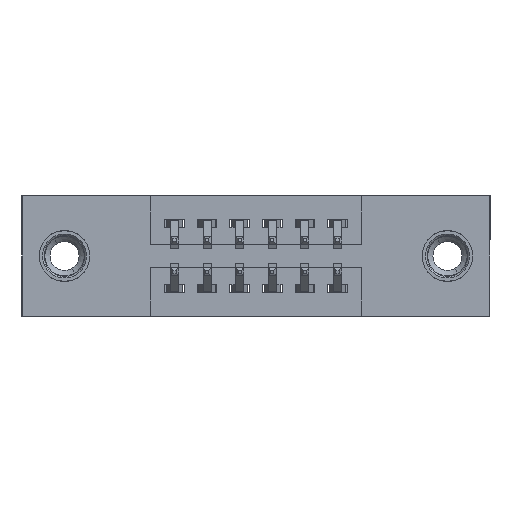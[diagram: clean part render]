
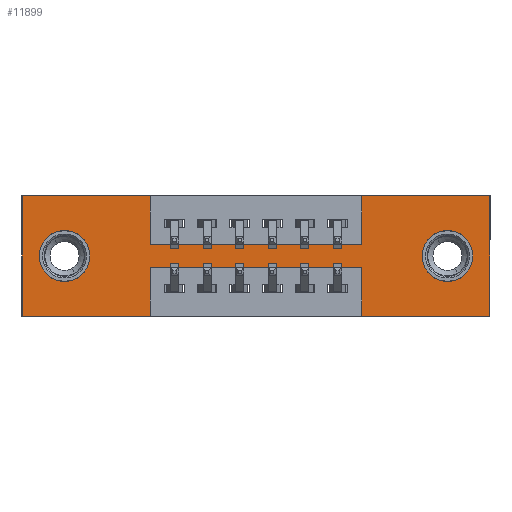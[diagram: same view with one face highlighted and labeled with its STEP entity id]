
A CAD part, front view. The second image highlights one B-rep face of the part: STEP entity #11899.
In plain terms, the highlighted planar face has unit normal (0, -1, 0).
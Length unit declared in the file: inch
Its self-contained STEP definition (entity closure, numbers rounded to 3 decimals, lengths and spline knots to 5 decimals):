
#12 = CARTESIAN_POINT ( 'NONE',  ( 1.0425, 0., -0.22 ) ) ;
#330 = DIRECTION ( 'NONE',  ( 0., -1., 0. ) ) ;
#574 = CARTESIAN_POINT ( 'NONE',  ( 0., 0., 0. ) ) ;
#660 = VECTOR ( 'NONE', #7857, 39.37008 ) ;
#666 = VERTEX_POINT ( 'NONE', #9988 ) ;
#913 = CARTESIAN_POINT ( 'NONE',  ( 0.13, 0., -0.185 ) ) ;
#924 = DIRECTION ( 'NONE',  ( -1., 0., 0. ) ) ;
#960 = EDGE_CURVE ( 'NONE', #5471, #2403, #10943, .T. ) ;
#980 = VERTEX_POINT ( 'NONE', #2272 ) ;
#1102 = EDGE_CURVE ( 'NONE', #11484, #6568, #4636, .T. ) ;
#1441 = DIRECTION ( 'NONE',  ( 0., 0., -1. ) ) ;
#1444 = VERTEX_POINT ( 'NONE', #6535 ) ;
#1849 = DIRECTION ( 'NONE',  ( 0., 0., 1. ) ) ;
#1892 = CARTESIAN_POINT ( 'NONE',  ( 0.3925, 0., -0.37 ) ) ;
#2001 = VECTOR ( 'NONE', #6488, 39.37008 ) ;
#2020 = CARTESIAN_POINT ( 'NONE',  ( 1.0425, 0., -0.37 ) ) ;
#2093 = ORIENTED_EDGE ( 'NONE', *, *, #5328, .F. ) ;
#2225 = EDGE_CURVE ( 'NONE', #10936, #7716, #7904, .T. ) ;
#2272 = CARTESIAN_POINT ( 'NONE',  ( 1.435, 0., 0. ) ) ;
#2368 = VECTOR ( 'NONE', #1441, 39.37008 ) ;
#2403 = VERTEX_POINT ( 'NONE', #3284 ) ;
#2464 = DIRECTION ( 'NONE',  ( 0., 0., 1. ) ) ;
#2514 = EDGE_CURVE ( 'NONE', #2403, #5872, #2651, .T. ) ;
#2546 = CARTESIAN_POINT ( 'NONE',  ( 0.3925, 0., -0.37 ) ) ;
#2635 = CARTESIAN_POINT ( 'NONE',  ( 1.0425, 0., 0. ) ) ;
#2651 = LINE ( 'NONE', #1892, #2368 ) ;
#2683 = CARTESIAN_POINT ( 'NONE',  ( 1.0425, 0., -0.37 ) ) ;
#2715 = AXIS2_PLACEMENT_3D ( 'NONE', #8161, #2724, #9088 ) ;
#2724 = DIRECTION ( 'NONE',  ( 0., 1., 0. ) ) ;
#2740 = EDGE_LOOP ( 'NONE', ( #7379, #7641, #11717, #3860, #4377, #10433, #2093, #8169, #8147, #10145, #6771, #6318 ) ) ;
#2841 = FACE_BOUND ( 'NONE', #7031, .T. ) ;
#2886 = CARTESIAN_POINT ( 'NONE',  ( 1.305, 0., -0.185 ) ) ;
#3093 = VECTOR ( 'NONE', #10019, 39.37008 ) ;
#3133 = LINE ( 'NONE', #9705, #660 ) ;
#3284 = CARTESIAN_POINT ( 'NONE',  ( 0.3925, 0., -0.22 ) ) ;
#3323 = CARTESIAN_POINT ( 'NONE',  ( 1.305, 0., -0.107 ) ) ;
#3369 = AXIS2_PLACEMENT_3D ( 'NONE', #913, #7292, #1849 ) ;
#3458 = EDGE_CURVE ( 'NONE', #10690, #666, #11189, .T. ) ;
#3465 = VERTEX_POINT ( 'NONE', #3323 ) ;
#3495 = CARTESIAN_POINT ( 'NONE',  ( 0., 0., 0. ) ) ;
#3556 = VECTOR ( 'NONE', #11845, 39.37008 ) ;
#3683 = DIRECTION ( 'NONE',  ( 1., 0., 0. ) ) ;
#3703 = ORIENTED_EDGE ( 'NONE', *, *, #6675, .T. ) ;
#3789 = DIRECTION ( 'NONE',  ( 0., 0., -1. ) ) ;
#3831 = VECTOR ( 'NONE', #11718, 39.37008 ) ;
#3860 = ORIENTED_EDGE ( 'NONE', *, *, #5424, .F. ) ;
#3888 = DIRECTION ( 'NONE',  ( 1., 0., 0. ) ) ;
#4115 = EDGE_CURVE ( 'NONE', #6568, #11484, #4578, .T. ) ;
#4146 = CARTESIAN_POINT ( 'NONE',  ( 0.3925, 0., -0.22 ) ) ;
#4232 = CIRCLE ( 'NONE', #10131, 0.078 ) ;
#4377 = ORIENTED_EDGE ( 'NONE', *, *, #4827, .F. ) ;
#4406 = DIRECTION ( 'NONE',  ( 0., 1., 0. ) ) ;
#4578 = CIRCLE ( 'NONE', #3369, 0.078 ) ;
#4636 = CIRCLE ( 'NONE', #6461, 0.078 ) ;
#4687 = LINE ( 'NONE', #5579, #6827 ) ;
#4827 = EDGE_CURVE ( 'NONE', #980, #8665, #4687, .T. ) ;
#4829 = EDGE_CURVE ( 'NONE', #5872, #5750, #9265, .T. ) ;
#4859 = ORIENTED_EDGE ( 'NONE', *, *, #4115, .T. ) ;
#4879 = LINE ( 'NONE', #10794, #11925 ) ;
#4903 = AXIS2_PLACEMENT_3D ( 'NONE', #11338, #330, #6755 ) ;
#4921 = PLANE ( 'NONE',  #4903 ) ;
#5164 = CARTESIAN_POINT ( 'NONE',  ( 1.0425, 0., -0.15 ) ) ;
#5190 = EDGE_CURVE ( 'NONE', #5750, #10690, #3133, .T. ) ;
#5328 = EDGE_CURVE ( 'NONE', #7716, #1444, #11125, .T. ) ;
#5424 = EDGE_CURVE ( 'NONE', #8665, #6189, #5680, .T. ) ;
#5471 = VERTEX_POINT ( 'NONE', #12 ) ;
#5537 = VERTEX_POINT ( 'NONE', #6556 ) ;
#5579 = CARTESIAN_POINT ( 'NONE',  ( 1.435, 0., 0. ) ) ;
#5584 = EDGE_CURVE ( 'NONE', #1444, #980, #6379, .T. ) ;
#5680 = LINE ( 'NONE', #11911, #7801 ) ;
#5750 = VERTEX_POINT ( 'NONE', #9641 ) ;
#5872 = VERTEX_POINT ( 'NONE', #2546 ) ;
#5961 = CIRCLE ( 'NONE', #2715, 0.078 ) ;
#6189 = VERTEX_POINT ( 'NONE', #2020 ) ;
#6318 = ORIENTED_EDGE ( 'NONE', *, *, #4829, .F. ) ;
#6378 = CARTESIAN_POINT ( 'NONE',  ( 0.3925, 0., -0.15 ) ) ;
#6379 = LINE ( 'NONE', #10298, #8532 ) ;
#6461 = AXIS2_PLACEMENT_3D ( 'NONE', #10319, #4406, #2464 ) ;
#6488 = DIRECTION ( 'NONE',  ( -1., 0., 0. ) ) ;
#6535 = CARTESIAN_POINT ( 'NONE',  ( 1.0425, 0., 0. ) ) ;
#6556 = CARTESIAN_POINT ( 'NONE',  ( 1.305, 0., -0.263 ) ) ;
#6568 = VERTEX_POINT ( 'NONE', #11851 ) ;
#6675 = EDGE_CURVE ( 'NONE', #3465, #5537, #4232, .T. ) ;
#6755 = DIRECTION ( 'NONE',  ( 0., 0., -1. ) ) ;
#6771 = ORIENTED_EDGE ( 'NONE', *, *, #5190, .F. ) ;
#6827 = VECTOR ( 'NONE', #10153, 39.37008 ) ;
#7031 = EDGE_LOOP ( 'NONE', ( #3703, #7633 ) ) ;
#7292 = DIRECTION ( 'NONE',  ( 0., 1., 0. ) ) ;
#7379 = ORIENTED_EDGE ( 'NONE', *, *, #2514, .F. ) ;
#7633 = ORIENTED_EDGE ( 'NONE', *, *, #11577, .T. ) ;
#7641 = ORIENTED_EDGE ( 'NONE', *, *, #960, .F. ) ;
#7672 = FACE_BOUND ( 'NONE', #9062, .T. ) ;
#7716 = VERTEX_POINT ( 'NONE', #5164 ) ;
#7801 = VECTOR ( 'NONE', #924, 39.37008 ) ;
#7857 = DIRECTION ( 'NONE',  ( 0., 0., 1. ) ) ;
#7904 = LINE ( 'NONE', #10504, #3093 ) ;
#8147 = ORIENTED_EDGE ( 'NONE', *, *, #9097, .F. ) ;
#8161 = CARTESIAN_POINT ( 'NONE',  ( 1.305, 0., -0.185 ) ) ;
#8169 = ORIENTED_EDGE ( 'NONE', *, *, #2225, .F. ) ;
#8211 = VECTOR ( 'NONE', #11298, 39.37008 ) ;
#8432 = CARTESIAN_POINT ( 'NONE',  ( 1.435, 0., -0.37 ) ) ;
#8532 = VECTOR ( 'NONE', #3888, 39.37008 ) ;
#8665 = VERTEX_POINT ( 'NONE', #8432 ) ;
#8690 = LINE ( 'NONE', #2683, #3556 ) ;
#8752 = VECTOR ( 'NONE', #3683, 39.37008 ) ;
#9062 = EDGE_LOOP ( 'NONE', ( #9939, #4859 ) ) ;
#9088 = DIRECTION ( 'NONE',  ( 0., 0., -1. ) ) ;
#9097 = EDGE_CURVE ( 'NONE', #666, #10936, #4879, .T. ) ;
#9250 = DIRECTION ( 'NONE',  ( 0., 1., 0. ) ) ;
#9265 = LINE ( 'NONE', #11055, #2001 ) ;
#9641 = CARTESIAN_POINT ( 'NONE',  ( 0., 0., -0.37 ) ) ;
#9705 = CARTESIAN_POINT ( 'NONE',  ( 0., 0., 0. ) ) ;
#9885 = DIRECTION ( 'NONE',  ( 0., 0., -1. ) ) ;
#9922 = CARTESIAN_POINT ( 'NONE',  ( 0.13, 0., -0.107 ) ) ;
#9939 = ORIENTED_EDGE ( 'NONE', *, *, #1102, .T. ) ;
#9988 = CARTESIAN_POINT ( 'NONE',  ( 0.3925, 0., 0. ) ) ;
#10019 = DIRECTION ( 'NONE',  ( 1., 0., 0. ) ) ;
#10130 = FACE_OUTER_BOUND ( 'NONE', #2740, .T. ) ;
#10131 = AXIS2_PLACEMENT_3D ( 'NONE', #2886, #9250, #3789 ) ;
#10145 = ORIENTED_EDGE ( 'NONE', *, *, #3458, .F. ) ;
#10153 = DIRECTION ( 'NONE',  ( 0., 0., -1. ) ) ;
#10298 = CARTESIAN_POINT ( 'NONE',  ( 0., 0., 0. ) ) ;
#10319 = CARTESIAN_POINT ( 'NONE',  ( 0.13, 0., -0.185 ) ) ;
#10433 = ORIENTED_EDGE ( 'NONE', *, *, #5584, .F. ) ;
#10504 = CARTESIAN_POINT ( 'NONE',  ( 0.3925, 0., -0.15 ) ) ;
#10690 = VERTEX_POINT ( 'NONE', #574 ) ;
#10794 = CARTESIAN_POINT ( 'NONE',  ( 0.3925, 0., 0. ) ) ;
#10936 = VERTEX_POINT ( 'NONE', #6378 ) ;
#10943 = LINE ( 'NONE', #4146, #8211 ) ;
#11055 = CARTESIAN_POINT ( 'NONE',  ( 0., 0., -0.37 ) ) ;
#11125 = LINE ( 'NONE', #2635, #3831 ) ;
#11189 = LINE ( 'NONE', #3495, #8752 ) ;
#11298 = DIRECTION ( 'NONE',  ( -1., 0., 0. ) ) ;
#11338 = CARTESIAN_POINT ( 'NONE',  ( 0., 0., -0.37 ) ) ;
#11484 = VERTEX_POINT ( 'NONE', #9922 ) ;
#11560 = EDGE_CURVE ( 'NONE', #6189, #5471, #8690, .T. ) ;
#11577 = EDGE_CURVE ( 'NONE', #5537, #3465, #5961, .T. ) ;
#11717 = ORIENTED_EDGE ( 'NONE', *, *, #11560, .F. ) ;
#11718 = DIRECTION ( 'NONE',  ( 0., 0., 1. ) ) ;
#11845 = DIRECTION ( 'NONE',  ( 0., 0., 1. ) ) ;
#11851 = CARTESIAN_POINT ( 'NONE',  ( 0.13, 0., -0.263 ) ) ;
#11899 = ADVANCED_FACE ( 'NONE', ( #2841, #7672, #10130 ), #4921, .T. ) ;
#11911 = CARTESIAN_POINT ( 'NONE',  ( 0., 0., -0.37 ) ) ;
#11925 = VECTOR ( 'NONE', #9885, 39.37008 ) ;
